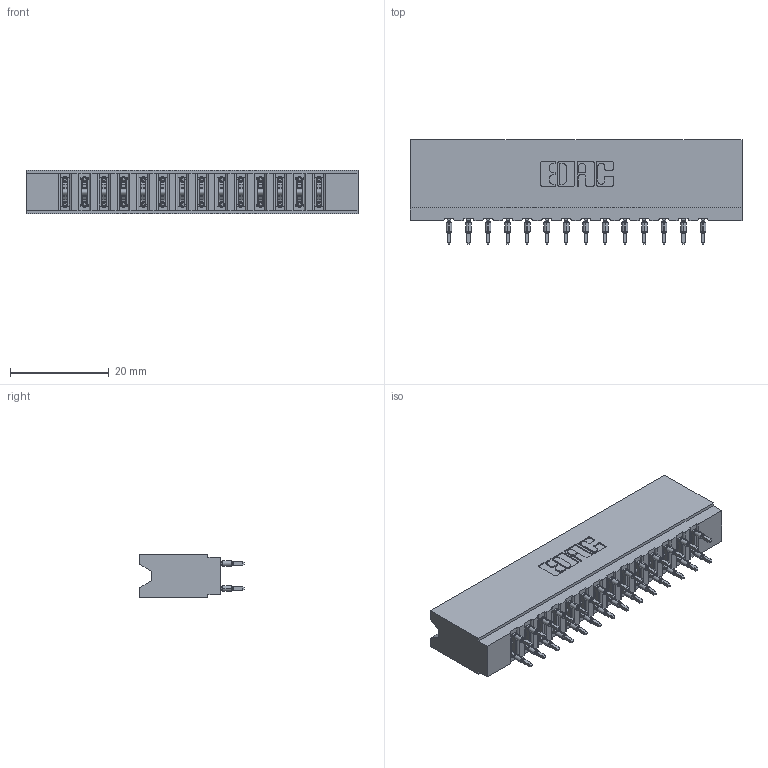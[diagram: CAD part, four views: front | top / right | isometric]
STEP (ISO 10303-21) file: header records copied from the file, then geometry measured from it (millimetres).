
FILE_DESCRIPTION (( 'STEP AP203' ), '1' );
FILE_NAME ('737-028-560-206.STEP', '2020-09-10T23:11:06', ( '' ), ( '' ), 'SwSTEP 2.0', 'SolidWorks 2020', '' );
FILE_SCHEMA (( 'CONFIG_CONTROL_DESIGN' ));
Length unit declared in the file: inch
Products named in the file (3): 737 Part_Insulator Option - 06; 745-292-001_560; 737-028-560-206
Assembly tree (29 placements, depth 2):
  737-028-560-206
    737 Part_Insulator Option - 06
    745-292-001_560  x28
Bounding box: 67.31 x 21.22 x 8.89 mm (x, y, z)
Volume: 6914.4 mm3; surface area: 9932.3 mm2
Topology: 29 solids, 29 shells, 2867 faces, 7845 edges, 4986 vertices
Faces by surface type: plane 1497, cylinder 642, bspline 560, torus 168
Entity records: 28170 total; most frequent: CARTESIAN_POINT 5402, ORIENTED_EDGE 4782, DIRECTION 4203, EDGE_CURVE 2391, LINE 2117, VECTOR 2117, VERTEX_POINT 1530, AXIS2_PLACEMENT_3D 1043
